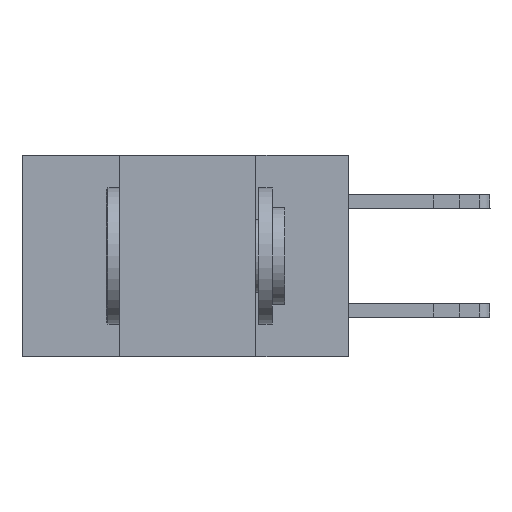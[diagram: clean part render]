
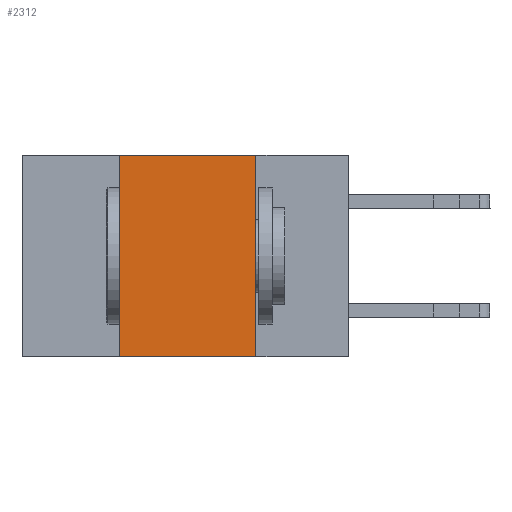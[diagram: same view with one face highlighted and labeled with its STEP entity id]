
A CAD part, left-side view. The second image highlights one B-rep face of the part: STEP entity #2312.
In plain terms, the highlighted planar face has unit normal (-1, 0, 0).
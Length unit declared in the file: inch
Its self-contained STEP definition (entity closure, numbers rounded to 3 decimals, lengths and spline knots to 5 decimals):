
#364 = EDGE_CURVE ( 'NONE', #6642, #4987, #9876, .T. ) ;
#403 = CARTESIAN_POINT ( 'NONE',  ( 0., 0.17, -0.37 ) ) ;
#744 = ORIENTED_EDGE ( 'NONE', *, *, #7183, .F. ) ;
#818 = EDGE_CURVE ( 'NONE', #4152, #1268, #12030, .T. ) ;
#1152 = ORIENTED_EDGE ( 'NONE', *, *, #364, .F. ) ;
#1268 = VERTEX_POINT ( 'NONE', #12940 ) ;
#1401 = LINE ( 'NONE', #403, #11337 ) ;
#1897 = ORIENTED_EDGE ( 'NONE', *, *, #9163, .F. ) ;
#2037 = CARTESIAN_POINT ( 'NONE',  ( 0., 0.6, -0.37 ) ) ;
#2312 = ADVANCED_FACE ( 'NONE', ( #6155 ), #14027, .F. ) ;
#2347 = VECTOR ( 'NONE', #6485, 39.37008 ) ;
#3779 = AXIS2_PLACEMENT_3D ( 'NONE', #10827, #4969, #9409 ) ;
#4152 = VERTEX_POINT ( 'NONE', #9948 ) ;
#4211 = LINE ( 'NONE', #12817, #9197 ) ;
#4813 = DIRECTION ( 'NONE',  ( 0., -1., 0. ) ) ;
#4816 = DIRECTION ( 'NONE',  ( 0., 0., -1. ) ) ;
#4969 = DIRECTION ( 'NONE',  ( 1., 0., 0. ) ) ;
#4987 = VERTEX_POINT ( 'NONE', #7665 ) ;
#5029 = CARTESIAN_POINT ( 'NONE',  ( 0., 0.42, 0. ) ) ;
#5172 = DIRECTION ( 'NONE',  ( 0., 0., 1. ) ) ;
#6155 = FACE_OUTER_BOUND ( 'NONE', #11620, .T. ) ;
#6485 = DIRECTION ( 'NONE',  ( 0., -1., 0. ) ) ;
#6642 = VERTEX_POINT ( 'NONE', #5029 ) ;
#7183 = EDGE_CURVE ( 'NONE', #4152, #6642, #4211, .T. ) ;
#7665 = CARTESIAN_POINT ( 'NONE',  ( 0., 0.17, 0. ) ) ;
#9163 = EDGE_CURVE ( 'NONE', #4987, #1268, #1401, .T. ) ;
#9197 = VECTOR ( 'NONE', #5172, 39.37008 ) ;
#9409 = DIRECTION ( 'NONE',  ( 0., 0., -1. ) ) ;
#9876 = LINE ( 'NONE', #13241, #13304 ) ;
#9948 = CARTESIAN_POINT ( 'NONE',  ( 0., 0.42, -0.37 ) ) ;
#10337 = ORIENTED_EDGE ( 'NONE', *, *, #818, .T. ) ;
#10827 = CARTESIAN_POINT ( 'NONE',  ( 0., 0.6, 0. ) ) ;
#11337 = VECTOR ( 'NONE', #4816, 39.37008 ) ;
#11620 = EDGE_LOOP ( 'NONE', ( #1897, #1152, #744, #10337 ) ) ;
#12030 = LINE ( 'NONE', #2037, #2347 ) ;
#12817 = CARTESIAN_POINT ( 'NONE',  ( 0., 0.42, -0.37 ) ) ;
#12940 = CARTESIAN_POINT ( 'NONE',  ( 0., 0.17, -0.37 ) ) ;
#13241 = CARTESIAN_POINT ( 'NONE',  ( 0., 0.6, 0. ) ) ;
#13304 = VECTOR ( 'NONE', #4813, 39.37008 ) ;
#14027 = PLANE ( 'NONE',  #3779 ) ;
